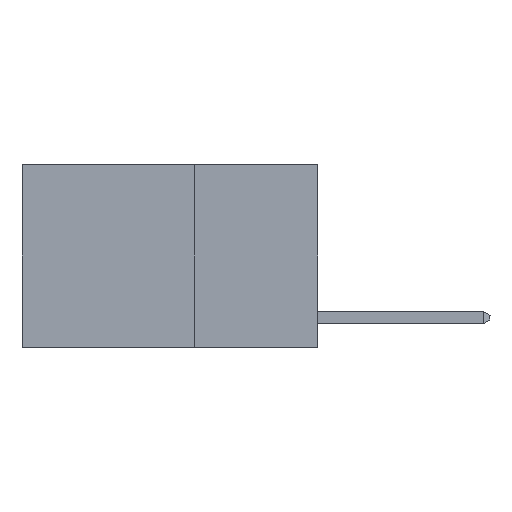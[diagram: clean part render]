
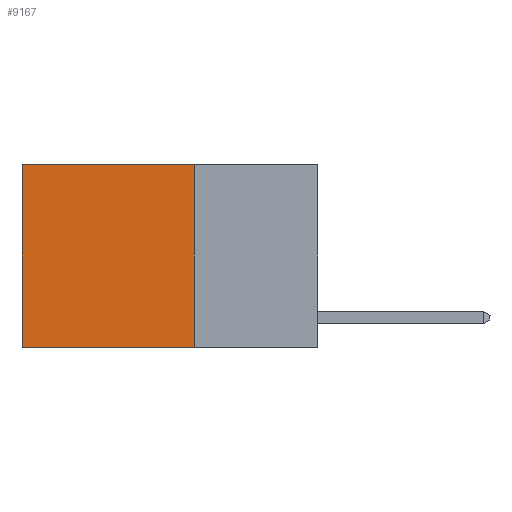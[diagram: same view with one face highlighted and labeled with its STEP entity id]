
A CAD part, left-side view. The second image highlights one B-rep face of the part: STEP entity #9167.
In plain terms, the highlighted planar face has unit normal (-1, 0, 0).
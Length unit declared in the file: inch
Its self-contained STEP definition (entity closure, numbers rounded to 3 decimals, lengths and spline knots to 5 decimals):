
#156 = VERTEX_POINT ( 'NONE', #6611 ) ;
#163 = EDGE_CURVE ( 'NONE', #1369, #156, #3330, .T. ) ;
#300 = FACE_OUTER_BOUND ( 'NONE', #9307, .T. ) ;
#478 = VECTOR ( 'NONE', #8992, 39.37008 ) ;
#576 = LINE ( 'NONE', #8070, #478 ) ;
#610 = ORIENTED_EDGE ( 'NONE', *, *, #10592, .F. ) ;
#675 = CARTESIAN_POINT ( 'NONE',  ( 0.2625, 0.25, -0.37 ) ) ;
#721 = DIRECTION ( 'NONE',  ( 0., 0., -1. ) ) ;
#917 = AXIS2_PLACEMENT_3D ( 'NONE', #6893, #6021, #6786 ) ;
#1238 = EDGE_CURVE ( 'NONE', #7624, #1369, #8132, .T. ) ;
#1369 = VERTEX_POINT ( 'NONE', #8519 ) ;
#1535 = ORIENTED_EDGE ( 'NONE', *, *, #1238, .T. ) ;
#1548 = CARTESIAN_POINT ( 'NONE',  ( 0.2625, 0.6, 0. ) ) ;
#1683 = EDGE_CURVE ( 'NONE', #7624, #9024, #6393, .T. ) ;
#2718 = PLANE ( 'NONE',  #917 ) ;
#3135 = CARTESIAN_POINT ( 'NONE',  ( 0.2625, 0.25, 0. ) ) ;
#3330 = LINE ( 'NONE', #1548, #3670 ) ;
#3670 = VECTOR ( 'NONE', #721, 39.37008 ) ;
#3706 = DIRECTION ( 'NONE',  ( 0., 0., -1. ) ) ;
#6021 = DIRECTION ( 'NONE',  ( 1., 0., 0. ) ) ;
#6163 = VECTOR ( 'NONE', #3706, 39.37008 ) ;
#6261 = DIRECTION ( 'NONE',  ( 0., 1., 0. ) ) ;
#6393 = LINE ( 'NONE', #7880, #6163 ) ;
#6611 = CARTESIAN_POINT ( 'NONE',  ( 0.2625, 0.6, -0.37 ) ) ;
#6786 = DIRECTION ( 'NONE',  ( 0., 0., -1. ) ) ;
#6893 = CARTESIAN_POINT ( 'NONE',  ( 0.2625, 0.25, 0. ) ) ;
#7500 = CARTESIAN_POINT ( 'NONE',  ( 0.2625, 0.25, 0. ) ) ;
#7536 = ORIENTED_EDGE ( 'NONE', *, *, #1683, .F. ) ;
#7624 = VERTEX_POINT ( 'NONE', #7500 ) ;
#7880 = CARTESIAN_POINT ( 'NONE',  ( 0.2625, 0.25, 0. ) ) ;
#8070 = CARTESIAN_POINT ( 'NONE',  ( 0.2625, 0.25, -0.37 ) ) ;
#8132 = LINE ( 'NONE', #3135, #9477 ) ;
#8519 = CARTESIAN_POINT ( 'NONE',  ( 0.2625, 0.6, 0. ) ) ;
#8992 = DIRECTION ( 'NONE',  ( 0., 1., 0. ) ) ;
#9024 = VERTEX_POINT ( 'NONE', #675 ) ;
#9167 = ADVANCED_FACE ( 'NONE', ( #300 ), #2718, .F. ) ;
#9307 = EDGE_LOOP ( 'NONE', ( #10705, #610, #7536, #1535 ) ) ;
#9477 = VECTOR ( 'NONE', #6261, 39.37008 ) ;
#10592 = EDGE_CURVE ( 'NONE', #9024, #156, #576, .T. ) ;
#10705 = ORIENTED_EDGE ( 'NONE', *, *, #163, .T. ) ;
